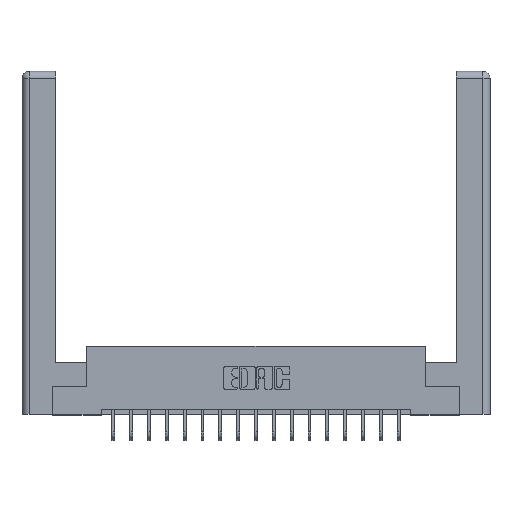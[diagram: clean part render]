
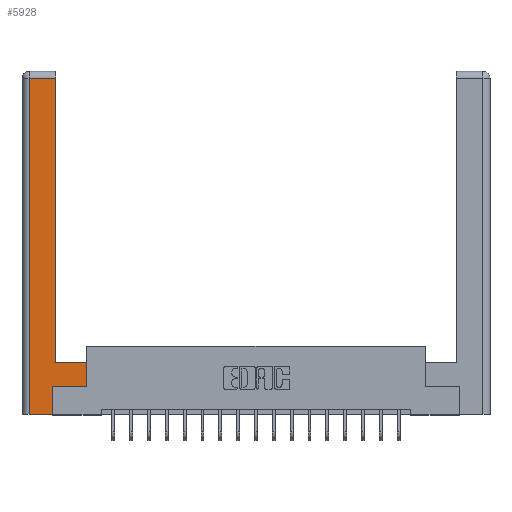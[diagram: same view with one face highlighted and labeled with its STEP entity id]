
A CAD part, top view. The second image highlights one B-rep face of the part: STEP entity #5928.
In plain terms, the highlighted planar face has unit normal (0, 0, 1).
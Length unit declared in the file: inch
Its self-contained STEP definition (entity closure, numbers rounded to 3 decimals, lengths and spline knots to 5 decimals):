
#484 = ORIENTED_EDGE ( 'NONE', *, *, #8097, .T. ) ;
#919 = CARTESIAN_POINT ( 'NONE',  ( 0.565, 0.45, 0. ) ) ;
#990 = CARTESIAN_POINT ( 'NONE',  ( 0.295, 0.45, 0. ) ) ;
#1085 = CARTESIAN_POINT ( 'NONE',  ( 0.565, 0.245, 0. ) ) ;
#1166 = ORIENTED_EDGE ( 'NONE', *, *, #4412, .T. ) ;
#1469 = DIRECTION ( 'NONE',  ( -1., 0., 0. ) ) ;
#1514 = VERTEX_POINT ( 'NONE', #14454 ) ;
#1979 = DIRECTION ( 'NONE',  ( 0., 1., 0. ) ) ;
#2280 = DIRECTION ( 'NONE',  ( 0., -1., 0. ) ) ;
#2465 = CARTESIAN_POINT ( 'NONE',  ( 0.265, 0., 0. ) ) ;
#2566 = VECTOR ( 'NONE', #2280, 39.37008 ) ;
#2688 = VECTOR ( 'NONE', #1979, 39.37008 ) ;
#2960 = LINE ( 'NONE', #6608, #8717 ) ;
#3040 = CARTESIAN_POINT ( 'NONE',  ( 0.565, 0.45, 0. ) ) ;
#3582 = LINE ( 'NONE', #16740, #2566 ) ;
#3839 = VERTEX_POINT ( 'NONE', #6425 ) ;
#3883 = EDGE_CURVE ( 'NONE', #17104, #9815, #8004, .T. ) ;
#4129 = EDGE_CURVE ( 'NONE', #3839, #13632, #7985, .T. ) ;
#4412 = EDGE_CURVE ( 'NONE', #9815, #20212, #2960, .T. ) ;
#5378 = CARTESIAN_POINT ( 'NONE',  ( 0.265, 0.245, 0. ) ) ;
#5413 = DIRECTION ( 'NONE',  ( 0., 1., 0. ) ) ;
#5461 = ORIENTED_EDGE ( 'NONE', *, *, #16573, .T. ) ;
#5928 = ADVANCED_FACE ( 'NONE', ( #14983 ), #17400, .F. ) ;
#6425 = CARTESIAN_POINT ( 'NONE',  ( 0.265, 0.245, 0. ) ) ;
#6560 = VECTOR ( 'NONE', #20477, 39.37008 ) ;
#6608 = CARTESIAN_POINT ( 'NONE',  ( 0.295, 3., 0. ) ) ;
#7985 = LINE ( 'NONE', #1085, #11047 ) ;
#8004 = LINE ( 'NONE', #11920, #14326 ) ;
#8097 = EDGE_CURVE ( 'NONE', #12996, #20326, #17928, .T. ) ;
#8346 = EDGE_CURVE ( 'NONE', #20212, #1514, #20345, .T. ) ;
#8717 = VECTOR ( 'NONE', #19485, 39.37008 ) ;
#9283 = CARTESIAN_POINT ( 'NONE',  ( 0.565, 0.245, 0. ) ) ;
#9593 = DIRECTION ( 'NONE',  ( 0., 0., -1. ) ) ;
#9815 = VERTEX_POINT ( 'NONE', #990 ) ;
#10256 = DIRECTION ( 'NONE',  ( -1., 0., 0. ) ) ;
#11047 = VECTOR ( 'NONE', #12419, 39.37008 ) ;
#11052 = CARTESIAN_POINT ( 'NONE',  ( 0., 0., 0. ) ) ;
#11590 = ORIENTED_EDGE ( 'NONE', *, *, #13469, .T. ) ;
#11920 = CARTESIAN_POINT ( 'NONE',  ( 0.295, 0.45, 0. ) ) ;
#12112 = CARTESIAN_POINT ( 'NONE',  ( 0.0615, 2.94, 0. ) ) ;
#12419 = DIRECTION ( 'NONE',  ( 1., 0., 0. ) ) ;
#12996 = VERTEX_POINT ( 'NONE', #14159 ) ;
#13069 = CARTESIAN_POINT ( 'NONE',  ( 0.265, 0., 0. ) ) ;
#13469 = EDGE_CURVE ( 'NONE', #1514, #12996, #3582, .T. ) ;
#13632 = VERTEX_POINT ( 'NONE', #9283 ) ;
#14159 = CARTESIAN_POINT ( 'NONE',  ( 0.0615, 0., 0. ) ) ;
#14201 = VECTOR ( 'NONE', #5413, 39.37008 ) ;
#14289 = ORIENTED_EDGE ( 'NONE', *, *, #4129, .T. ) ;
#14326 = VECTOR ( 'NONE', #10256, 39.37008 ) ;
#14454 = CARTESIAN_POINT ( 'NONE',  ( 0.0615, 2.94, 0. ) ) ;
#14889 = ORIENTED_EDGE ( 'NONE', *, *, #3883, .T. ) ;
#14983 = FACE_OUTER_BOUND ( 'NONE', #17162, .T. ) ;
#15363 = DIRECTION ( 'NONE',  ( -1., 0., 0. ) ) ;
#16573 = EDGE_CURVE ( 'NONE', #20326, #3839, #19352, .T. ) ;
#16740 = CARTESIAN_POINT ( 'NONE',  ( 0.0615, 0., 0. ) ) ;
#17104 = VERTEX_POINT ( 'NONE', #3040 ) ;
#17162 = EDGE_LOOP ( 'NONE', ( #1166, #20199, #11590, #484, #5461, #14289, #18812, #14889 ) ) ;
#17233 = AXIS2_PLACEMENT_3D ( 'NONE', #11052, #9593, #1469 ) ;
#17400 = PLANE ( 'NONE',  #17233 ) ;
#17928 = LINE ( 'NONE', #2465, #6560 ) ;
#18527 = EDGE_CURVE ( 'NONE', #13632, #17104, #20028, .T. ) ;
#18812 = ORIENTED_EDGE ( 'NONE', *, *, #18527, .T. ) ;
#19247 = CARTESIAN_POINT ( 'NONE',  ( 0.295, 2.94, 0. ) ) ;
#19352 = LINE ( 'NONE', #5378, #2688 ) ;
#19485 = DIRECTION ( 'NONE',  ( 0., 1., 0. ) ) ;
#20028 = LINE ( 'NONE', #919, #14201 ) ;
#20199 = ORIENTED_EDGE ( 'NONE', *, *, #8346, .T. ) ;
#20212 = VERTEX_POINT ( 'NONE', #19247 ) ;
#20319 = VECTOR ( 'NONE', #15363, 39.37008 ) ;
#20326 = VERTEX_POINT ( 'NONE', #13069 ) ;
#20345 = LINE ( 'NONE', #12112, #20319 ) ;
#20477 = DIRECTION ( 'NONE',  ( 1., 0., 0. ) ) ;
